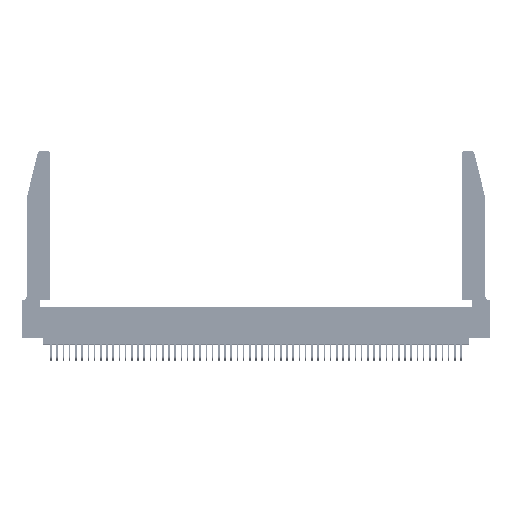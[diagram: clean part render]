
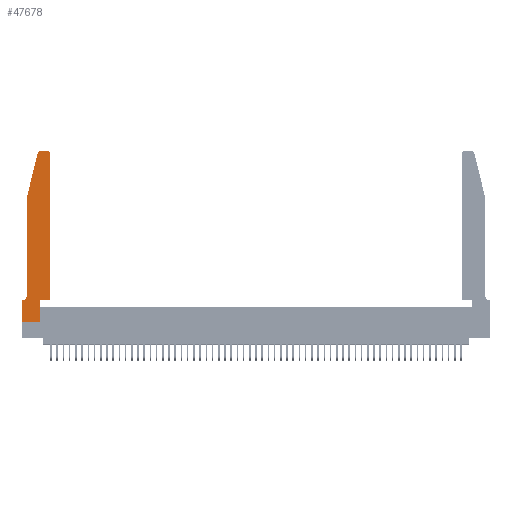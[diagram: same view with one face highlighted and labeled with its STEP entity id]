
A CAD part, top view. The second image highlights one B-rep face of the part: STEP entity #47678.
In plain terms, the highlighted planar face has unit normal (0, 0, 1).
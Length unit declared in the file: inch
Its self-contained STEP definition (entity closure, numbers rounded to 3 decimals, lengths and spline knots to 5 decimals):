
#279 = VERTEX_POINT ( 'NONE', #36281 ) ;
#295 = ORIENTED_EDGE ( 'NONE', *, *, #23375, .T. ) ;
#471 = DIRECTION ( 'NONE',  ( -0.239, -0.971, 0. ) ) ;
#1004 = LINE ( 'NONE', #3732, #46059 ) ;
#1984 = VECTOR ( 'NONE', #37654, 39.37008 ) ;
#2101 = CARTESIAN_POINT ( 'NONE',  ( 0.284, 2.75, 0.37 ) ) ;
#2161 = CARTESIAN_POINT ( 'NONE',  ( 0.0755, 2., 0.37 ) ) ;
#2173 = LINE ( 'NONE', #39036, #20298 ) ;
#2851 = AXIS2_PLACEMENT_3D ( 'NONE', #5282, #52314, #22423 ) ;
#3416 = ORIENTED_EDGE ( 'NONE', *, *, #4483, .T. ) ;
#3711 = CIRCLE ( 'NONE', #2851, 0.03 ) ;
#3732 = CARTESIAN_POINT ( 'NONE',  ( 0.4505, 0.35, 0.37 ) ) ;
#4410 = EDGE_CURVE ( 'NONE', #40134, #24568, #12807, .T. ) ;
#4483 = EDGE_CURVE ( 'NONE', #36355, #27418, #12045, .T. ) ;
#4829 = EDGE_CURVE ( 'NONE', #22088, #35202, #1004, .T. ) ;
#5282 = CARTESIAN_POINT ( 'NONE',  ( 0.4205, 2.72, 0.37 ) ) ;
#6409 = ORIENTED_EDGE ( 'NONE', *, *, #15260, .T. ) ;
#6510 = CARTESIAN_POINT ( 'NONE',  ( 0., 0., 0.37 ) ) ;
#6512 = ORIENTED_EDGE ( 'NONE', *, *, #4829, .T. ) ;
#6519 = CARTESIAN_POINT ( 'NONE',  ( 0.0755, 0.42, 0.37 ) ) ;
#6907 = VERTEX_POINT ( 'NONE', #17301 ) ;
#6930 = ORIENTED_EDGE ( 'NONE', *, *, #4410, .T. ) ;
#6955 = CARTESIAN_POINT ( 'NONE',  ( 0.0755, 2., 0.37 ) ) ;
#7370 = VECTOR ( 'NONE', #16182, 39.37008 ) ;
#7708 = CARTESIAN_POINT ( 'NONE',  ( 0.4205, 2.75, 0.37 ) ) ;
#8129 = CARTESIAN_POINT ( 'NONE',  ( 0.4505, 0.35, 0.37 ) ) ;
#8182 = VECTOR ( 'NONE', #40365, 39.37008 ) ;
#11344 = DIRECTION ( 'NONE',  ( -1., 0., 0. ) ) ;
#11448 = ORIENTED_EDGE ( 'NONE', *, *, #35823, .T. ) ;
#11987 = DIRECTION ( 'NONE',  ( -1., 0., 0. ) ) ;
#12045 = CIRCLE ( 'NONE', #44114, 0.07 ) ;
#12807 = CIRCLE ( 'NONE', #18185, 0.03 ) ;
#13031 = ORIENTED_EDGE ( 'NONE', *, *, #21393, .T. ) ;
#13706 = VERTEX_POINT ( 'NONE', #7708 ) ;
#15260 = EDGE_CURVE ( 'NONE', #35202, #279, #24368, .T. ) ;
#15984 = DIRECTION ( 'NONE',  ( 1., 0., 0. ) ) ;
#16182 = DIRECTION ( 'NONE',  ( 0., -1., 0. ) ) ;
#16936 = ORIENTED_EDGE ( 'NONE', *, *, #35700, .T. ) ;
#16990 = VERTEX_POINT ( 'NONE', #52399 ) ;
#17279 = CARTESIAN_POINT ( 'NONE',  ( 0.2865, 0.35, 0.37 ) ) ;
#17301 = CARTESIAN_POINT ( 'NONE',  ( 0., 0., 0.37 ) ) ;
#18185 = AXIS2_PLACEMENT_3D ( 'NONE', #52881, #26753, #44206 ) ;
#18407 = CARTESIAN_POINT ( 'NONE',  ( 0.0055, 0.35, 0.37 ) ) ;
#18526 = VECTOR ( 'NONE', #26777, 39.37008 ) ;
#20298 = VECTOR ( 'NONE', #471, 39.37008 ) ;
#21056 = EDGE_CURVE ( 'NONE', #27418, #29698, #47475, .T. ) ;
#21105 = CARTESIAN_POINT ( 'NONE',  ( 0.4505, 0.35, 0.37 ) ) ;
#21393 = EDGE_CURVE ( 'NONE', #279, #13706, #3711, .T. ) ;
#21407 = DIRECTION ( 'NONE',  ( 1., 0., 0. ) ) ;
#22088 = VERTEX_POINT ( 'NONE', #17279 ) ;
#22423 = DIRECTION ( 'NONE',  ( 1., 0., 0. ) ) ;
#23003 = VECTOR ( 'NONE', #55575, 39.37008 ) ;
#23375 = EDGE_CURVE ( 'NONE', #6907, #16990, #45194, .T. ) ;
#24053 = CARTESIAN_POINT ( 'NONE',  ( 0., 0.35, 0.37 ) ) ;
#24368 = LINE ( 'NONE', #8129, #23003 ) ;
#24568 = VERTEX_POINT ( 'NONE', #31450 ) ;
#24833 = PLANE ( 'NONE',  #43275 ) ;
#26069 = EDGE_LOOP ( 'NONE', ( #33820, #6930, #38470, #16936, #3416, #42819, #11448, #295, #53404, #6512, #6409, #13031 ) ) ;
#26753 = DIRECTION ( 'NONE',  ( 0., 0., 1. ) ) ;
#26777 = DIRECTION ( 'NONE',  ( 0., 1., 0. ) ) ;
#27290 = DIRECTION ( 'NONE',  ( 0., 0., -1. ) ) ;
#27418 = VERTEX_POINT ( 'NONE', #18407 ) ;
#29698 = VERTEX_POINT ( 'NONE', #24053 ) ;
#30032 = VECTOR ( 'NONE', #11344, 39.37008 ) ;
#31450 = CARTESIAN_POINT ( 'NONE',  ( 0.25487, 2.72718, 0.37 ) ) ;
#32350 = CARTESIAN_POINT ( 'NONE',  ( 0., 0.35, 0.37 ) ) ;
#33805 = CARTESIAN_POINT ( 'NONE',  ( 0.2605, 2.75, 0.37 ) ) ;
#33820 = ORIENTED_EDGE ( 'NONE', *, *, #50503, .T. ) ;
#34873 = CARTESIAN_POINT ( 'NONE',  ( 0.2865, 0.35, 0.37 ) ) ;
#35202 = VERTEX_POINT ( 'NONE', #21105 ) ;
#35700 = EDGE_CURVE ( 'NONE', #39433, #36355, #55178, .T. ) ;
#35823 = EDGE_CURVE ( 'NONE', #29698, #6907, #43691, .T. ) ;
#36281 = CARTESIAN_POINT ( 'NONE',  ( 0.4505, 2.72, 0.37 ) ) ;
#36355 = VERTEX_POINT ( 'NONE', #6519 ) ;
#37654 = DIRECTION ( 'NONE',  ( 0., -1., 0. ) ) ;
#37853 = EDGE_CURVE ( 'NONE', #16990, #22088, #51503, .T. ) ;
#38260 = FACE_OUTER_BOUND ( 'NONE', #26069, .T. ) ;
#38470 = ORIENTED_EDGE ( 'NONE', *, *, #52587, .T. ) ;
#39036 = CARTESIAN_POINT ( 'NONE',  ( 0.0755, 2., 0.37 ) ) ;
#39433 = VERTEX_POINT ( 'NONE', #2161 ) ;
#40134 = VERTEX_POINT ( 'NONE', #2101 ) ;
#40365 = DIRECTION ( 'NONE',  ( 1., 0., 0. ) ) ;
#40791 = LINE ( 'NONE', #33805, #41443 ) ;
#40968 = DIRECTION ( 'NONE',  ( 0., 0., 1. ) ) ;
#41443 = VECTOR ( 'NONE', #11987, 39.37008 ) ;
#41920 = CARTESIAN_POINT ( 'NONE',  ( 0., 0., 0.37 ) ) ;
#42819 = ORIENTED_EDGE ( 'NONE', *, *, #21056, .T. ) ;
#43275 = AXIS2_PLACEMENT_3D ( 'NONE', #32350, #40968, #15984 ) ;
#43691 = LINE ( 'NONE', #41920, #7370 ) ;
#44114 = AXIS2_PLACEMENT_3D ( 'NONE', #53064, #27290, #48531 ) ;
#44206 = DIRECTION ( 'NONE',  ( 1., 0., 0. ) ) ;
#45194 = LINE ( 'NONE', #6510, #8182 ) ;
#46059 = VECTOR ( 'NONE', #21407, 39.37008 ) ;
#47475 = LINE ( 'NONE', #55203, #30032 ) ;
#47678 = ADVANCED_FACE ( 'NONE', ( #38260 ), #24833, .T. ) ;
#48531 = DIRECTION ( 'NONE',  ( -1., 0., 0. ) ) ;
#50503 = EDGE_CURVE ( 'NONE', #13706, #40134, #40791, .T. ) ;
#51503 = LINE ( 'NONE', #34873, #18526 ) ;
#52314 = DIRECTION ( 'NONE',  ( 0., 0., 1. ) ) ;
#52399 = CARTESIAN_POINT ( 'NONE',  ( 0.2865, 0., 0.37 ) ) ;
#52587 = EDGE_CURVE ( 'NONE', #24568, #39433, #2173, .T. ) ;
#52881 = CARTESIAN_POINT ( 'NONE',  ( 0.284, 2.72, 0.37 ) ) ;
#53064 = CARTESIAN_POINT ( 'NONE',  ( 0.0055, 0.42, 0.37 ) ) ;
#53404 = ORIENTED_EDGE ( 'NONE', *, *, #37853, .T. ) ;
#55178 = LINE ( 'NONE', #6955, #1984 ) ;
#55203 = CARTESIAN_POINT ( 'NONE',  ( 0.0755, 0.35, 0.37 ) ) ;
#55575 = DIRECTION ( 'NONE',  ( 0., 1., 0. ) ) ;
